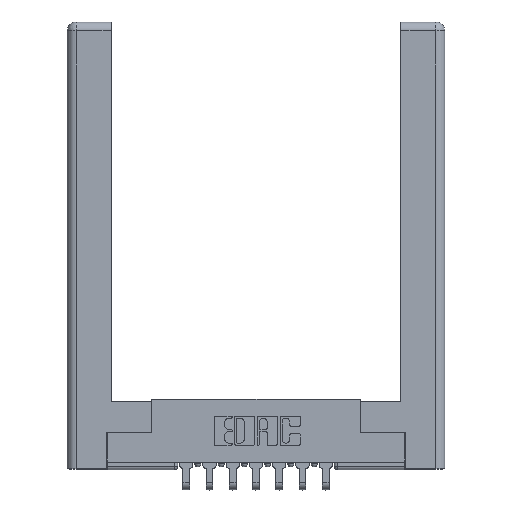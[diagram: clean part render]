
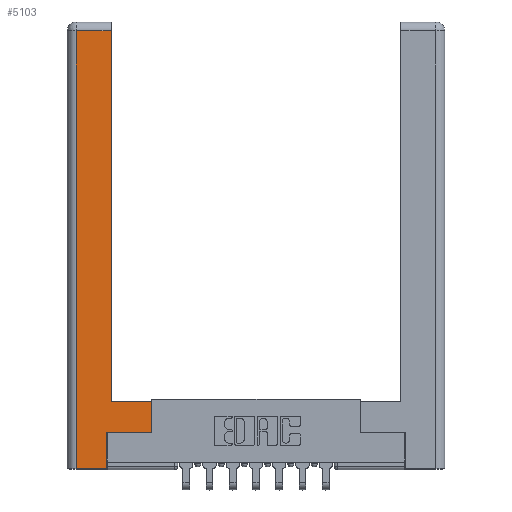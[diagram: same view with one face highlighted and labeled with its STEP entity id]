
A CAD part, top view. The second image highlights one B-rep face of the part: STEP entity #5103.
In plain terms, the highlighted planar face has unit normal (0, 0, 1).
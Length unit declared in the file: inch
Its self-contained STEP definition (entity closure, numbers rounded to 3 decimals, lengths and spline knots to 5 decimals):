
#106 = LINE ( 'NONE', #3857, #4211 ) ;
#122 = DIRECTION ( 'NONE',  ( 0., -1., 0. ) ) ;
#271 = CARTESIAN_POINT ( 'NONE',  ( 0.565, 0.45, 0. ) ) ;
#293 = DIRECTION ( 'NONE',  ( 1., 0., 0. ) ) ;
#773 = ORIENTED_EDGE ( 'NONE', *, *, #10115, .T. ) ;
#774 = CARTESIAN_POINT ( 'NONE',  ( 0.565, 0.45, 0. ) ) ;
#864 = VERTEX_POINT ( 'NONE', #11131 ) ;
#1730 = DIRECTION ( 'NONE',  ( -1., 0., 0. ) ) ;
#1908 = CARTESIAN_POINT ( 'NONE',  ( 0.565, 0.245, 0. ) ) ;
#2338 = VERTEX_POINT ( 'NONE', #3030 ) ;
#2405 = DIRECTION ( 'NONE',  ( 1., 0., 0. ) ) ;
#2654 = VECTOR ( 'NONE', #7918, 39.37008 ) ;
#2692 = ORIENTED_EDGE ( 'NONE', *, *, #12370, .T. ) ;
#2974 = ORIENTED_EDGE ( 'NONE', *, *, #5395, .T. ) ;
#3030 = CARTESIAN_POINT ( 'NONE',  ( 0.0615, 0., 0. ) ) ;
#3134 = AXIS2_PLACEMENT_3D ( 'NONE', #11813, #6821, #1730 ) ;
#3257 = CARTESIAN_POINT ( 'NONE',  ( 0.265, 0., 0. ) ) ;
#3314 = ORIENTED_EDGE ( 'NONE', *, *, #11285, .T. ) ;
#3749 = PLANE ( 'NONE',  #3134 ) ;
#3857 = CARTESIAN_POINT ( 'NONE',  ( 0.295, 3., 0. ) ) ;
#3866 = VECTOR ( 'NONE', #293, 39.37008 ) ;
#3969 = VECTOR ( 'NONE', #4821, 39.37008 ) ;
#4211 = VECTOR ( 'NONE', #10831, 39.37008 ) ;
#4393 = VERTEX_POINT ( 'NONE', #9587 ) ;
#4813 = LINE ( 'NONE', #13011, #7066 ) ;
#4821 = DIRECTION ( 'NONE',  ( -1., 0., 0. ) ) ;
#4854 = VERTEX_POINT ( 'NONE', #9331 ) ;
#4869 = EDGE_CURVE ( 'NONE', #7545, #8432, #8863, .T. ) ;
#4885 = CARTESIAN_POINT ( 'NONE',  ( 0.265, 0.245, 0. ) ) ;
#4892 = FACE_OUTER_BOUND ( 'NONE', #8984, .T. ) ;
#4949 = DIRECTION ( 'NONE',  ( -1., 0., 0. ) ) ;
#5064 = ORIENTED_EDGE ( 'NONE', *, *, #7855, .T. ) ;
#5103 = ADVANCED_FACE ( 'NONE', ( #4892 ), #3749, .F. ) ;
#5395 = EDGE_CURVE ( 'NONE', #4393, #7545, #9004, .T. ) ;
#5599 = ORIENTED_EDGE ( 'NONE', *, *, #8612, .T. ) ;
#5722 = LINE ( 'NONE', #12786, #3969 ) ;
#6140 = ORIENTED_EDGE ( 'NONE', *, *, #7637, .T. ) ;
#6798 = LINE ( 'NONE', #4885, #2654 ) ;
#6821 = DIRECTION ( 'NONE',  ( 0., 0., -1. ) ) ;
#7066 = VECTOR ( 'NONE', #4949, 39.37008 ) ;
#7545 = VERTEX_POINT ( 'NONE', #1908 ) ;
#7637 = EDGE_CURVE ( 'NONE', #2338, #10501, #12703, .T. ) ;
#7855 = EDGE_CURVE ( 'NONE', #12885, #864, #4813, .T. ) ;
#7918 = DIRECTION ( 'NONE',  ( 0., 1., 0. ) ) ;
#7937 = CARTESIAN_POINT ( 'NONE',  ( 0.295, 2.94, 0. ) ) ;
#8432 = VERTEX_POINT ( 'NONE', #774 ) ;
#8496 = CARTESIAN_POINT ( 'NONE',  ( 0.565, 0.245, 0. ) ) ;
#8544 = ORIENTED_EDGE ( 'NONE', *, *, #4869, .T. ) ;
#8612 = EDGE_CURVE ( 'NONE', #8432, #4854, #5722, .T. ) ;
#8707 = LINE ( 'NONE', #10141, #11202 ) ;
#8863 = LINE ( 'NONE', #271, #12942 ) ;
#8953 = CARTESIAN_POINT ( 'NONE',  ( 0.265, 0., 0. ) ) ;
#8984 = EDGE_LOOP ( 'NONE', ( #2692, #5064, #773, #6140, #3314, #2974, #8544, #5599 ) ) ;
#9004 = LINE ( 'NONE', #8496, #9152 ) ;
#9152 = VECTOR ( 'NONE', #2405, 39.37008 ) ;
#9331 = CARTESIAN_POINT ( 'NONE',  ( 0.295, 0.45, 0. ) ) ;
#9587 = CARTESIAN_POINT ( 'NONE',  ( 0.265, 0.245, 0. ) ) ;
#10115 = EDGE_CURVE ( 'NONE', #864, #2338, #8707, .T. ) ;
#10141 = CARTESIAN_POINT ( 'NONE',  ( 0.0615, 0., 0. ) ) ;
#10501 = VERTEX_POINT ( 'NONE', #8953 ) ;
#10831 = DIRECTION ( 'NONE',  ( 0., 1., 0. ) ) ;
#11131 = CARTESIAN_POINT ( 'NONE',  ( 0.0615, 2.94, 0. ) ) ;
#11202 = VECTOR ( 'NONE', #122, 39.37008 ) ;
#11285 = EDGE_CURVE ( 'NONE', #10501, #4393, #6798, .T. ) ;
#11813 = CARTESIAN_POINT ( 'NONE',  ( 0., 0., 0. ) ) ;
#12370 = EDGE_CURVE ( 'NONE', #4854, #12885, #106, .T. ) ;
#12478 = DIRECTION ( 'NONE',  ( 0., 1., 0. ) ) ;
#12703 = LINE ( 'NONE', #3257, #3866 ) ;
#12786 = CARTESIAN_POINT ( 'NONE',  ( 0.295, 0.45, 0. ) ) ;
#12885 = VERTEX_POINT ( 'NONE', #7937 ) ;
#12942 = VECTOR ( 'NONE', #12478, 39.37008 ) ;
#13011 = CARTESIAN_POINT ( 'NONE',  ( 0.0615, 2.94, 0. ) ) ;
